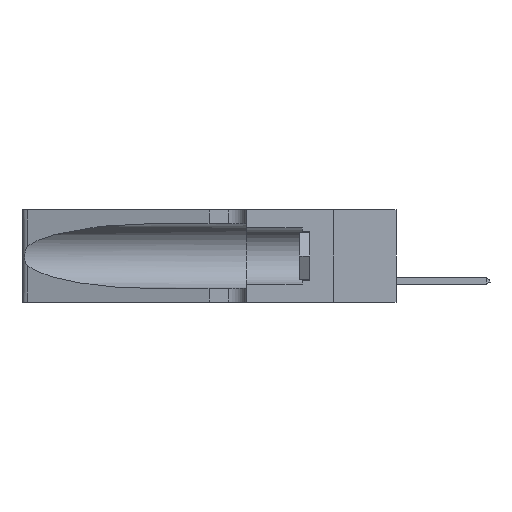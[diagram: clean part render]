
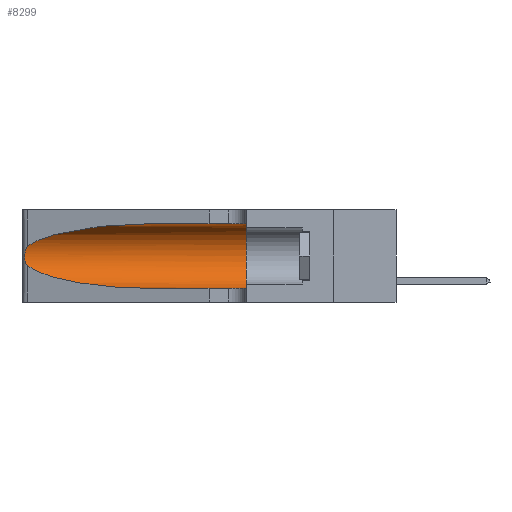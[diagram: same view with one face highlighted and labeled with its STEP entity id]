
A CAD part, left-side view. The second image highlights one B-rep face of the part: STEP entity #8299.
In plain terms, the highlighted cylindrical face has radius 3.308 mm (diameter 6.617 mm), a partial arc.
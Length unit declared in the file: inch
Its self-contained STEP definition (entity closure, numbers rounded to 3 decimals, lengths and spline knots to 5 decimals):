
#414 = FACE_OUTER_BOUND ( 'NONE', #2450, .T. ) ;
#802 = EDGE_CURVE ( 'NONE', #18553, #22193, #9906, .T. ) ;
#1230 = DIRECTION ( 'NONE',  ( 0., -1., 0. ) ) ;
#1499 = CARTESIAN_POINT ( 'NONE',  ( 0.25487, 1.22718, 0.14631 ) ) ;
#1681 = DIRECTION ( 'NONE',  ( 0., 1., 0. ) ) ;
#2450 = EDGE_LOOP ( 'NONE', ( #6844, #23134, #7555, #13013, #13962, #22205 ) ) ;
#2676 = CARTESIAN_POINT ( 'NONE',  ( 0.25856, 1.23593, 0.16098 ) ) ;
#2919 = CARTESIAN_POINT ( 'NONE',  ( 0.2373, 1.15595, 0.28018 ) ) ;
#3010 = CARTESIAN_POINT ( 'NONE',  ( 0.25639, 1.23184, 0.21858 ) ) ;
#3044 = VERTEX_POINT ( 'NONE', #21346 ) ;
#4108 = VERTEX_POINT ( 'NONE', #7455 ) ;
#4151 = DIRECTION ( 'NONE',  ( 0., 0., -1. ) ) ;
#6477 = CARTESIAN_POINT ( 'NONE',  ( 0.18966, 0.96281, 0.31525 ) ) ;
#6719 =( BOUNDED_CURVE ( )  B_SPLINE_CURVE ( 3, ( #22459, #11224, #22294, #17588 ),
 .UNSPECIFIED., .F., .F. ) 
 B_SPLINE_CURVE_WITH_KNOTS ( ( 4, 4 ),
 ( 3.44316, 4.71239 ),
 .UNSPECIFIED. ) 
 CURVE ( )  GEOMETRIC_REPRESENTATION_ITEM ( )  RATIONAL_B_SPLINE_CURVE ( ( 1., 0.87, 0.87, 1. ) ) 
 REPRESENTATION_ITEM ( '' )  );
#6822 = CARTESIAN_POINT ( 'NONE',  ( 0.25854, 1.2359, 0.20912 ) ) ;
#6844 = ORIENTED_EDGE ( 'NONE', *, *, #13510, .T. ) ;
#6988 = VERTEX_POINT ( 'NONE', #8362 ) ;
#7455 = CARTESIAN_POINT ( 'NONE',  ( 0.1305, 0.72297, 0.31525 ) ) ;
#7555 = ORIENTED_EDGE ( 'NONE', *, *, #7787, .T. ) ;
#7582 = AXIS2_PLACEMENT_3D ( 'NONE', #22462, #1681, #20780 ) ;
#7780 =( BOUNDED_CURVE ( )  B_SPLINE_CURVE ( 3, ( #10362, #6477, #2919, #23593 ),
 .UNSPECIFIED., .F., .F. ) 
 B_SPLINE_CURVE_WITH_KNOTS ( ( 4, 4 ),
 ( 1.5708, 2.84003 ),
 .UNSPECIFIED. ) 
 CURVE ( )  GEOMETRIC_REPRESENTATION_ITEM ( )  RATIONAL_B_SPLINE_CURVE ( ( 1., 0.87, 0.87, 1. ) ) 
 REPRESENTATION_ITEM ( '' )  );
#7787 = EDGE_CURVE ( 'NONE', #22193, #22012, #6719, .T. ) ;
#8299 = ADVANCED_FACE ( 'NONE', ( #414 ), #9043, .F. ) ;
#8362 = CARTESIAN_POINT ( 'NONE',  ( 0.1305, 0.35, 0.31525 ) ) ;
#8707 = CARTESIAN_POINT ( 'NONE',  ( 0.26075, 1.23896, 0.19203 ) ) ;
#9043 = CYLINDRICAL_SURFACE ( 'NONE', #19169, 0.13025 ) ;
#9906 = B_SPLINE_CURVE_WITH_KNOTS ( 'NONE', 3,
 ( #12268, #21769, #3010, #18098, #6822, #20033, #8707, #10624, #12516, #2676, #23514, #12186, #11049, #1499 ),
 .UNSPECIFIED., .F., .F.,
 ( 4, 2, 2, 2, 2, 2, 4 ),
 ( 0., 0.00027, 0.00053, 0.00107, 0.0016, 0.00187, 0.00214 ),
 .UNSPECIFIED. ) ;
#10362 = CARTESIAN_POINT ( 'NONE',  ( 0.1305, 0.72297, 0.31525 ) ) ;
#10578 = VECTOR ( 'NONE', #1230, 39.37008 ) ;
#10624 = CARTESIAN_POINT ( 'NONE',  ( 0.26075, 1.23896, 0.178 ) ) ;
#10801 = CARTESIAN_POINT ( 'NONE',  ( 0.25487, 1.22718, 0.14631 ) ) ;
#11034 = CARTESIAN_POINT ( 'NONE',  ( 0.25487, 1.22718, 0.22369 ) ) ;
#11049 = CARTESIAN_POINT ( 'NONE',  ( 0.25555, 1.22993, 0.14849 ) ) ;
#11224 = CARTESIAN_POINT ( 'NONE',  ( 0.2373, 1.15595, 0.08982 ) ) ;
#11364 = CARTESIAN_POINT ( 'NONE',  ( 0.1305, 1.61858, 0.185 ) ) ;
#11652 = LINE ( 'NONE', #24307, #11929 ) ;
#11929 = VECTOR ( 'NONE', #18660, 39.37008 ) ;
#12186 = CARTESIAN_POINT ( 'NONE',  ( 0.25639, 1.23186, 0.15144 ) ) ;
#12268 = CARTESIAN_POINT ( 'NONE',  ( 0.25487, 1.22718, 0.22369 ) ) ;
#12516 = CARTESIAN_POINT ( 'NONE',  ( 0.26017, 1.23833, 0.17102 ) ) ;
#13013 = ORIENTED_EDGE ( 'NONE', *, *, #23787, .T. ) ;
#13510 = EDGE_CURVE ( 'NONE', #4108, #18553, #7780, .T. ) ;
#13962 = ORIENTED_EDGE ( 'NONE', *, *, #23313, .F. ) ;
#14737 = CARTESIAN_POINT ( 'NONE',  ( 0.1305, 1.61858, 0.05475 ) ) ;
#15766 = EDGE_CURVE ( 'NONE', #4108, #6988, #11652, .T. ) ;
#17283 = CIRCLE ( 'NONE', #7582, 0.13025 ) ;
#17588 = CARTESIAN_POINT ( 'NONE',  ( 0.1305, 0.72297, 0.05475 ) ) ;
#18098 = CARTESIAN_POINT ( 'NONE',  ( 0.25787, 1.23484, 0.2124 ) ) ;
#18553 = VERTEX_POINT ( 'NONE', #11034 ) ;
#18660 = DIRECTION ( 'NONE',  ( 0., -1., 0. ) ) ;
#19111 = CARTESIAN_POINT ( 'NONE',  ( 0.1305, 0.72297, 0.05475 ) ) ;
#19169 = AXIS2_PLACEMENT_3D ( 'NONE', #11364, #22765, #4151 ) ;
#20033 = CARTESIAN_POINT ( 'NONE',  ( 0.26018, 1.23835, 0.19895 ) ) ;
#20780 = DIRECTION ( 'NONE',  ( 0., 0., 1. ) ) ;
#21346 = CARTESIAN_POINT ( 'NONE',  ( 0.1305, 0.35, 0.05475 ) ) ;
#21769 = CARTESIAN_POINT ( 'NONE',  ( 0.25555, 1.22994, 0.2215 ) ) ;
#22012 = VERTEX_POINT ( 'NONE', #19111 ) ;
#22193 = VERTEX_POINT ( 'NONE', #10801 ) ;
#22205 = ORIENTED_EDGE ( 'NONE', *, *, #15766, .F. ) ;
#22294 = CARTESIAN_POINT ( 'NONE',  ( 0.18966, 0.96281, 0.05475 ) ) ;
#22459 = CARTESIAN_POINT ( 'NONE',  ( 0.25487, 1.22718, 0.14631 ) ) ;
#22462 = CARTESIAN_POINT ( 'NONE',  ( 0.1305, 0.35, 0.185 ) ) ;
#22765 = DIRECTION ( 'NONE',  ( 0., -1., 0. ) ) ;
#23134 = ORIENTED_EDGE ( 'NONE', *, *, #802, .T. ) ;
#23313 = EDGE_CURVE ( 'NONE', #6988, #3044, #17283, .T. ) ;
#23514 = CARTESIAN_POINT ( 'NONE',  ( 0.25789, 1.23486, 0.15765 ) ) ;
#23579 = LINE ( 'NONE', #14737, #10578 ) ;
#23593 = CARTESIAN_POINT ( 'NONE',  ( 0.25487, 1.22718, 0.22369 ) ) ;
#23787 = EDGE_CURVE ( 'NONE', #22012, #3044, #23579, .T. ) ;
#24307 = CARTESIAN_POINT ( 'NONE',  ( 0.1305, 1.61858, 0.31525 ) ) ;
